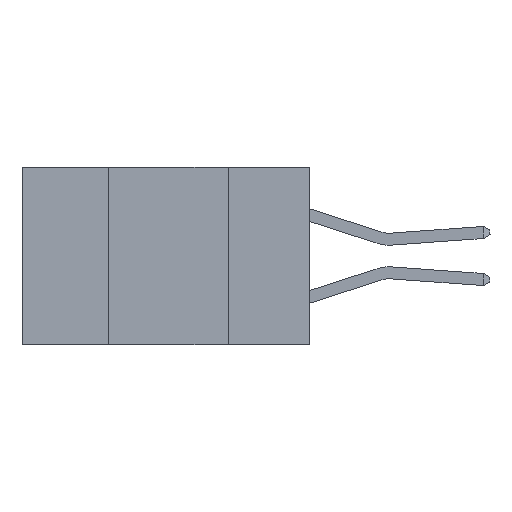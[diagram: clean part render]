
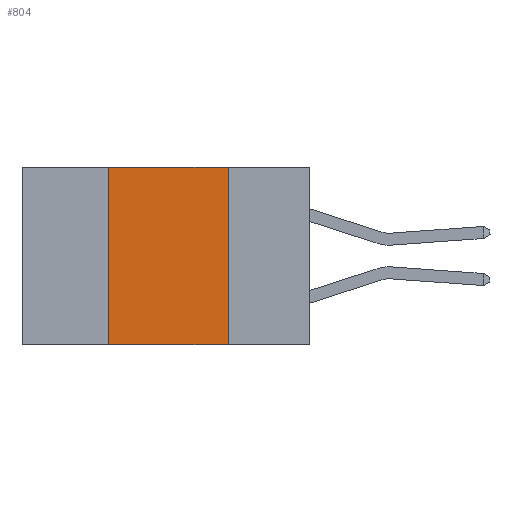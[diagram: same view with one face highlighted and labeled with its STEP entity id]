
A CAD part, left-side view. The second image highlights one B-rep face of the part: STEP entity #804.
In plain terms, the highlighted planar face has unit normal (-1, 0, 0).
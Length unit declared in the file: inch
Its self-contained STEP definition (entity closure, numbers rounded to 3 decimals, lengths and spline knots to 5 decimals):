
#144 = CARTESIAN_POINT ( 'NONE',  ( 0., 0.42, -0.37 ) ) ;
#804 = ADVANCED_FACE ( 'NONE', ( #7541 ), #7483, .F. ) ;
#1671 = LINE ( 'NONE', #144, #5396 ) ;
#1711 = ORIENTED_EDGE ( 'NONE', *, *, #4069, .F. ) ;
#1896 = DIRECTION ( 'NONE',  ( 0., 0., -1. ) ) ;
#2046 = VECTOR ( 'NONE', #5852, 39.37008 ) ;
#2344 = AXIS2_PLACEMENT_3D ( 'NONE', #6572, #9008, #1896 ) ;
#2555 = CARTESIAN_POINT ( 'NONE',  ( 0., 0.17, 0. ) ) ;
#2596 = LINE ( 'NONE', #6537, #2046 ) ;
#3413 = DIRECTION ( 'NONE',  ( 0., 0., 1. ) ) ;
#3532 = VERTEX_POINT ( 'NONE', #10436 ) ;
#4003 = EDGE_LOOP ( 'NONE', ( #7976, #7784, #1711, #6394 ) ) ;
#4069 = EDGE_CURVE ( 'NONE', #7246, #3532, #1671, .T. ) ;
#4691 = EDGE_CURVE ( 'NONE', #7577, #5349, #5167, .T. ) ;
#5132 = EDGE_CURVE ( 'NONE', #7246, #5349, #8374, .T. ) ;
#5167 = LINE ( 'NONE', #5331, #8605 ) ;
#5331 = CARTESIAN_POINT ( 'NONE',  ( 0., 0.17, -0.37 ) ) ;
#5349 = VERTEX_POINT ( 'NONE', #7867 ) ;
#5396 = VECTOR ( 'NONE', #3413, 39.37008 ) ;
#5852 = DIRECTION ( 'NONE',  ( 0., -1., 0. ) ) ;
#5976 = CARTESIAN_POINT ( 'NONE',  ( 0., 0.42, -0.37 ) ) ;
#6394 = ORIENTED_EDGE ( 'NONE', *, *, #5132, .T. ) ;
#6537 = CARTESIAN_POINT ( 'NONE',  ( 0., 0.6, 0. ) ) ;
#6572 = CARTESIAN_POINT ( 'NONE',  ( 0., 0.6, 0. ) ) ;
#6695 = DIRECTION ( 'NONE',  ( 0., -1., 0. ) ) ;
#6761 = VECTOR ( 'NONE', #6695, 39.37008 ) ;
#6812 = DIRECTION ( 'NONE',  ( 0., 0., -1. ) ) ;
#7246 = VERTEX_POINT ( 'NONE', #5976 ) ;
#7483 = PLANE ( 'NONE',  #2344 ) ;
#7541 = FACE_OUTER_BOUND ( 'NONE', #4003, .T. ) ;
#7577 = VERTEX_POINT ( 'NONE', #2555 ) ;
#7784 = ORIENTED_EDGE ( 'NONE', *, *, #9280, .F. ) ;
#7867 = CARTESIAN_POINT ( 'NONE',  ( 0., 0.17, -0.37 ) ) ;
#7976 = ORIENTED_EDGE ( 'NONE', *, *, #4691, .F. ) ;
#8374 = LINE ( 'NONE', #8533, #6761 ) ;
#8533 = CARTESIAN_POINT ( 'NONE',  ( 0., 0.6, -0.37 ) ) ;
#8605 = VECTOR ( 'NONE', #6812, 39.37008 ) ;
#9008 = DIRECTION ( 'NONE',  ( 1., 0., 0. ) ) ;
#9280 = EDGE_CURVE ( 'NONE', #3532, #7577, #2596, .T. ) ;
#10436 = CARTESIAN_POINT ( 'NONE',  ( 0., 0.42, 0. ) ) ;
